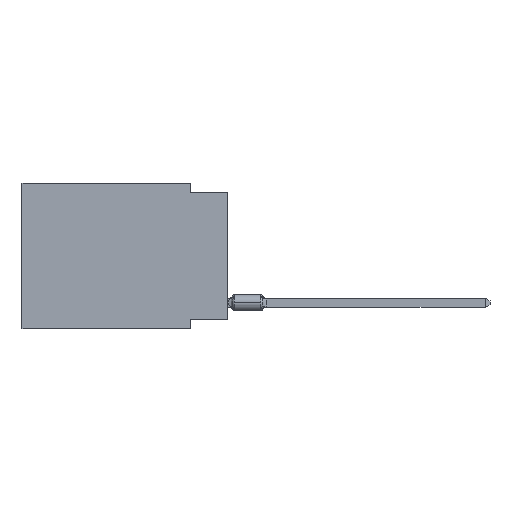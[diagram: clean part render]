
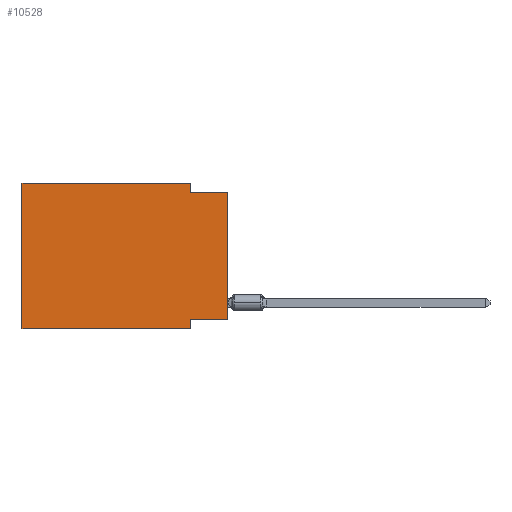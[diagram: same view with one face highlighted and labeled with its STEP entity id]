
A CAD part, left-side view. The second image highlights one B-rep face of the part: STEP entity #10528.
In plain terms, the highlighted planar face has unit normal (-1, 0, 0).
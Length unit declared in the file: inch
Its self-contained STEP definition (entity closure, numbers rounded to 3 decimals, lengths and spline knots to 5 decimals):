
#303 = ORIENTED_EDGE ( 'NONE', *, *, #13186, .F. ) ;
#485 = ORIENTED_EDGE ( 'NONE', *, *, #11010, .T. ) ;
#1107 = CARTESIAN_POINT ( 'NONE',  ( 0., 0.1, -0.365 ) ) ;
#1433 = LINE ( 'NONE', #4522, #18506 ) ;
#1523 = VERTEX_POINT ( 'NONE', #3691 ) ;
#2098 = LINE ( 'NONE', #15983, #18389 ) ;
#2333 = CARTESIAN_POINT ( 'NONE',  ( 0., 0.1, -0.39 ) ) ;
#2745 = ORIENTED_EDGE ( 'NONE', *, *, #6618, .F. ) ;
#3344 = CARTESIAN_POINT ( 'NONE',  ( 0., 0.1, -0.025 ) ) ;
#3432 = ORIENTED_EDGE ( 'NONE', *, *, #12128, .F. ) ;
#3691 = CARTESIAN_POINT ( 'NONE',  ( 0., 0., -0.365 ) ) ;
#4101 = EDGE_CURVE ( 'NONE', #1523, #16869, #5204, .T. ) ;
#4107 = VECTOR ( 'NONE', #12628, 39.37008 ) ;
#4138 = VECTOR ( 'NONE', #11044, 39.37008 ) ;
#4235 = CARTESIAN_POINT ( 'NONE',  ( 0., 0.1, 0. ) ) ;
#4522 = CARTESIAN_POINT ( 'NONE',  ( 0., 0., -0.025 ) ) ;
#4673 = FACE_OUTER_BOUND ( 'NONE', #13758, .T. ) ;
#4918 = VERTEX_POINT ( 'NONE', #3344 ) ;
#5152 = AXIS2_PLACEMENT_3D ( 'NONE', #6451, #13882, #12212 ) ;
#5204 = LINE ( 'NONE', #15619, #4107 ) ;
#5371 = EDGE_CURVE ( 'NONE', #9286, #15534, #14222, .T. ) ;
#5377 = VECTOR ( 'NONE', #19094, 39.37008 ) ;
#5665 = EDGE_CURVE ( 'NONE', #13022, #4918, #2098, .T. ) ;
#5859 = DIRECTION ( 'NONE',  ( 0., 0., 1. ) ) ;
#6288 = DIRECTION ( 'NONE',  ( 0., 0., 1. ) ) ;
#6451 = CARTESIAN_POINT ( 'NONE',  ( 0., 0.55, 0. ) ) ;
#6618 = EDGE_CURVE ( 'NONE', #16869, #15534, #15920, .T. ) ;
#6666 = EDGE_CURVE ( 'NONE', #12872, #13022, #7270, .T. ) ;
#7174 = DIRECTION ( 'NONE',  ( 0., -1., 0. ) ) ;
#7270 = LINE ( 'NONE', #17679, #10748 ) ;
#8379 = CARTESIAN_POINT ( 'NONE',  ( 0., 0.55, -0.39 ) ) ;
#9286 = VERTEX_POINT ( 'NONE', #18526 ) ;
#9730 = DIRECTION ( 'NONE',  ( 0., 0., -1. ) ) ;
#9867 = ORIENTED_EDGE ( 'NONE', *, *, #5371, .T. ) ;
#10528 = ADVANCED_FACE ( 'NONE', ( #4673 ), #18350, .F. ) ;
#10748 = VECTOR ( 'NONE', #7174, 39.37008 ) ;
#11010 = EDGE_CURVE ( 'NONE', #1523, #16311, #16272, .T. ) ;
#11036 = ORIENTED_EDGE ( 'NONE', *, *, #4101, .F. ) ;
#11044 = DIRECTION ( 'NONE',  ( 0., -1., 0. ) ) ;
#11243 = LINE ( 'NONE', #12739, #15950 ) ;
#12128 = EDGE_CURVE ( 'NONE', #9286, #12872, #11243, .T. ) ;
#12212 = DIRECTION ( 'NONE',  ( 0., 0., -1. ) ) ;
#12562 = CARTESIAN_POINT ( 'NONE',  ( 0., 0.55, 0. ) ) ;
#12628 = DIRECTION ( 'NONE',  ( 0., 1., 0. ) ) ;
#12739 = CARTESIAN_POINT ( 'NONE',  ( 0., 0.55, 0. ) ) ;
#12865 = CARTESIAN_POINT ( 'NONE',  ( 0., 0., -0.025 ) ) ;
#12872 = VERTEX_POINT ( 'NONE', #12562 ) ;
#13022 = VERTEX_POINT ( 'NONE', #4235 ) ;
#13186 = EDGE_CURVE ( 'NONE', #4918, #16311, #1433, .T. ) ;
#13635 = DIRECTION ( 'NONE',  ( 0., -1., 0. ) ) ;
#13758 = EDGE_LOOP ( 'NONE', ( #485, #303, #14106, #16712, #3432, #9867, #2745, #11036 ) ) ;
#13882 = DIRECTION ( 'NONE',  ( 1., 0., 0. ) ) ;
#14106 = ORIENTED_EDGE ( 'NONE', *, *, #5665, .F. ) ;
#14222 = LINE ( 'NONE', #8379, #4138 ) ;
#14512 = CARTESIAN_POINT ( 'NONE',  ( 0., 0.1, -0.39 ) ) ;
#14988 = CARTESIAN_POINT ( 'NONE',  ( 0., 0., 0. ) ) ;
#15534 = VERTEX_POINT ( 'NONE', #14512 ) ;
#15619 = CARTESIAN_POINT ( 'NONE',  ( 0., 0., -0.365 ) ) ;
#15920 = LINE ( 'NONE', #2333, #5377 ) ;
#15950 = VECTOR ( 'NONE', #6288, 39.37008 ) ;
#15983 = CARTESIAN_POINT ( 'NONE',  ( 0., 0.1, 0. ) ) ;
#16272 = LINE ( 'NONE', #14988, #16867 ) ;
#16311 = VERTEX_POINT ( 'NONE', #12865 ) ;
#16712 = ORIENTED_EDGE ( 'NONE', *, *, #6666, .F. ) ;
#16867 = VECTOR ( 'NONE', #5859, 39.37008 ) ;
#16869 = VERTEX_POINT ( 'NONE', #1107 ) ;
#17679 = CARTESIAN_POINT ( 'NONE',  ( 0., 0.55, 0. ) ) ;
#18350 = PLANE ( 'NONE',  #5152 ) ;
#18389 = VECTOR ( 'NONE', #9730, 39.37008 ) ;
#18506 = VECTOR ( 'NONE', #13635, 39.37008 ) ;
#18526 = CARTESIAN_POINT ( 'NONE',  ( 0., 0.55, -0.39 ) ) ;
#19094 = DIRECTION ( 'NONE',  ( 0., 0., -1. ) ) ;
